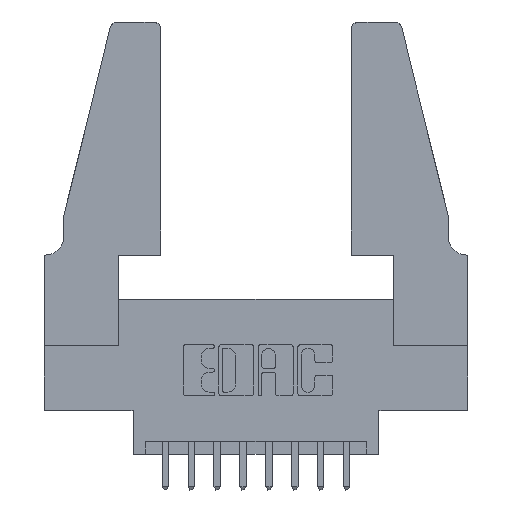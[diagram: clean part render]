
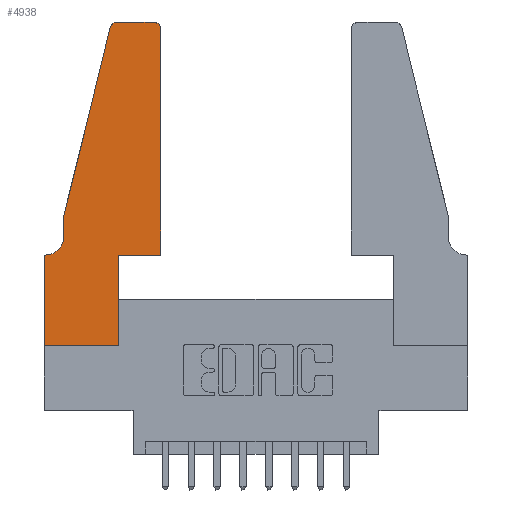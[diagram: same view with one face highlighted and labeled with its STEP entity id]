
A CAD part, top view. The second image highlights one B-rep face of the part: STEP entity #4938.
In plain terms, the highlighted planar face has unit normal (0, 0, 1).
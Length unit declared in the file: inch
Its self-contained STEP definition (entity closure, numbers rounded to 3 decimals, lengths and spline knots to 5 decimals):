
#205 = CARTESIAN_POINT ( 'NONE',  ( 0.284, 1.22, 0.37 ) ) ;
#284 = DIRECTION ( 'NONE',  ( 0., 0., 1. ) ) ;
#294 = EDGE_CURVE ( 'NONE', #1931, #2083, #7622, .T. ) ;
#692 = DIRECTION ( 'NONE',  ( 0., 1., 0. ) ) ;
#739 = CARTESIAN_POINT ( 'NONE',  ( 0.0755, 0.5, 0.37 ) ) ;
#795 = CARTESIAN_POINT ( 'NONE',  ( 0.0755, 0.42, 0.37 ) ) ;
#846 = EDGE_CURVE ( 'NONE', #7038, #6351, #1083, .T. ) ;
#870 = DIRECTION ( 'NONE',  ( 1., 0., 0. ) ) ;
#997 = ORIENTED_EDGE ( 'NONE', *, *, #3256, .T. ) ;
#1051 = CARTESIAN_POINT ( 'NONE',  ( 0.0755, 0.5, 0.37 ) ) ;
#1083 = LINE ( 'NONE', #8374, #8864 ) ;
#1498 = DIRECTION ( 'NONE',  ( 1., 0., 0. ) ) ;
#1621 = DIRECTION ( 'NONE',  ( 0., 0., -1. ) ) ;
#1684 = CARTESIAN_POINT ( 'NONE',  ( 0.0755, 0.35, 0.37 ) ) ;
#1690 = DIRECTION ( 'NONE',  ( 0., -1., 0. ) ) ;
#1698 = DIRECTION ( 'NONE',  ( -1., 0., 0. ) ) ;
#1899 = CIRCLE ( 'NONE', #6041, 0.07 ) ;
#1931 = VERTEX_POINT ( 'NONE', #13122 ) ;
#2083 = VERTEX_POINT ( 'NONE', #4257 ) ;
#2161 = AXIS2_PLACEMENT_3D ( 'NONE', #11984, #6101, #870 ) ;
#2348 = DIRECTION ( 'NONE',  ( 1., 0., 0. ) ) ;
#2449 = CARTESIAN_POINT ( 'NONE',  ( 0.4205, 1.22, 0.37 ) ) ;
#2551 = CARTESIAN_POINT ( 'NONE',  ( 0., 0., 0.37 ) ) ;
#2644 = CARTESIAN_POINT ( 'NONE',  ( 0.0055, 0.42, 0.37 ) ) ;
#2874 = DIRECTION ( 'NONE',  ( -1., 0., 0. ) ) ;
#3157 = VERTEX_POINT ( 'NONE', #10702 ) ;
#3256 = EDGE_CURVE ( 'NONE', #11287, #6496, #10385, .T. ) ;
#3401 = EDGE_LOOP ( 'NONE', ( #11480, #9987, #997, #12524, #6514, #8560, #8275, #5488, #4520, #5731, #10199, #4979 ) ) ;
#3553 = CARTESIAN_POINT ( 'NONE',  ( 0.4505, 0.35, 0.37 ) ) ;
#3646 = EDGE_CURVE ( 'NONE', #5559, #4359, #5180, .T. ) ;
#4061 = PLANE ( 'NONE',  #2161 ) ;
#4157 = EDGE_CURVE ( 'NONE', #4359, #12903, #7979, .T. ) ;
#4257 = CARTESIAN_POINT ( 'NONE',  ( 0., 0.35, 0.37 ) ) ;
#4306 = VECTOR ( 'NONE', #10437, 39.37008 ) ;
#4350 = DIRECTION ( 'NONE',  ( 0., 0., 1. ) ) ;
#4359 = VERTEX_POINT ( 'NONE', #11068 ) ;
#4520 = ORIENTED_EDGE ( 'NONE', *, *, #4157, .T. ) ;
#4556 = LINE ( 'NONE', #1051, #11165 ) ;
#4602 = CARTESIAN_POINT ( 'NONE',  ( 0.4505, 0.35, 0.37 ) ) ;
#4938 = ADVANCED_FACE ( 'NONE', ( #8599 ), #4061, .T. ) ;
#4979 = ORIENTED_EDGE ( 'NONE', *, *, #6165, .T. ) ;
#5180 = LINE ( 'NONE', #11621, #12761 ) ;
#5488 = ORIENTED_EDGE ( 'NONE', *, *, #3646, .T. ) ;
#5559 = VERTEX_POINT ( 'NONE', #2551 ) ;
#5731 = ORIENTED_EDGE ( 'NONE', *, *, #7010, .T. ) ;
#5947 = VECTOR ( 'NONE', #1698, 39.37008 ) ;
#5952 = VECTOR ( 'NONE', #692, 39.37008 ) ;
#6041 = AXIS2_PLACEMENT_3D ( 'NONE', #2644, #1621, #7700 ) ;
#6101 = DIRECTION ( 'NONE',  ( 0., 0., 1. ) ) ;
#6165 = EDGE_CURVE ( 'NONE', #6351, #3157, #9343, .T. ) ;
#6251 = CARTESIAN_POINT ( 'NONE',  ( 0.2865, 0.35, 0.37 ) ) ;
#6351 = VERTEX_POINT ( 'NONE', #12873 ) ;
#6447 = DIRECTION ( 'NONE',  ( 0., -1., 0. ) ) ;
#6496 = VERTEX_POINT ( 'NONE', #13127 ) ;
#6514 = ORIENTED_EDGE ( 'NONE', *, *, #7148, .T. ) ;
#6743 = CARTESIAN_POINT ( 'NONE',  ( 0.284, 1.25, 0.37 ) ) ;
#6774 = CARTESIAN_POINT ( 'NONE',  ( 0.2605, 1.25, 0.37 ) ) ;
#7010 = EDGE_CURVE ( 'NONE', #12903, #7038, #9349, .T. ) ;
#7038 = VERTEX_POINT ( 'NONE', #4602 ) ;
#7148 = EDGE_CURVE ( 'NONE', #10518, #1931, #1899, .T. ) ;
#7197 = LINE ( 'NONE', #6774, #5947 ) ;
#7273 = AXIS2_PLACEMENT_3D ( 'NONE', #2449, #284, #2348 ) ;
#7422 = DIRECTION ( 'NONE',  ( 1., 0., 0. ) ) ;
#7469 = VECTOR ( 'NONE', #2874, 39.37008 ) ;
#7542 = VECTOR ( 'NONE', #8811, 39.37008 ) ;
#7622 = LINE ( 'NONE', #1684, #7469 ) ;
#7700 = DIRECTION ( 'NONE',  ( -1., 0., 0. ) ) ;
#7863 = EDGE_CURVE ( 'NONE', #2083, #5559, #11432, .T. ) ;
#7979 = LINE ( 'NONE', #13042, #5952 ) ;
#8070 = VECTOR ( 'NONE', #1690, 39.37008 ) ;
#8082 = CIRCLE ( 'NONE', #13096, 0.03 ) ;
#8175 = EDGE_CURVE ( 'NONE', #6496, #10518, #4556, .T. ) ;
#8275 = ORIENTED_EDGE ( 'NONE', *, *, #7863, .T. ) ;
#8374 = CARTESIAN_POINT ( 'NONE',  ( 0.4505, 0.35, 0.37 ) ) ;
#8560 = ORIENTED_EDGE ( 'NONE', *, *, #294, .T. ) ;
#8599 = FACE_OUTER_BOUND ( 'NONE', #3401, .T. ) ;
#8692 = CARTESIAN_POINT ( 'NONE',  ( 0., 0., 0.37 ) ) ;
#8811 = DIRECTION ( 'NONE',  ( -0.239, -0.971, 0. ) ) ;
#8864 = VECTOR ( 'NONE', #10014, 39.37008 ) ;
#8895 = EDGE_CURVE ( 'NONE', #3157, #12568, #7197, .T. ) ;
#9343 = CIRCLE ( 'NONE', #7273, 0.03 ) ;
#9349 = LINE ( 'NONE', #3553, #4306 ) ;
#9987 = ORIENTED_EDGE ( 'NONE', *, *, #10200, .T. ) ;
#10014 = DIRECTION ( 'NONE',  ( 0., 1., 0. ) ) ;
#10199 = ORIENTED_EDGE ( 'NONE', *, *, #846, .T. ) ;
#10200 = EDGE_CURVE ( 'NONE', #12568, #11287, #8082, .T. ) ;
#10385 = LINE ( 'NONE', #739, #7542 ) ;
#10437 = DIRECTION ( 'NONE',  ( 1., 0., 0. ) ) ;
#10518 = VERTEX_POINT ( 'NONE', #795 ) ;
#10702 = CARTESIAN_POINT ( 'NONE',  ( 0.4205, 1.25, 0.37 ) ) ;
#11068 = CARTESIAN_POINT ( 'NONE',  ( 0.2865, 0., 0.37 ) ) ;
#11165 = VECTOR ( 'NONE', #6447, 39.37008 ) ;
#11287 = VERTEX_POINT ( 'NONE', #11469 ) ;
#11432 = LINE ( 'NONE', #8692, #8070 ) ;
#11469 = CARTESIAN_POINT ( 'NONE',  ( 0.25487, 1.22718, 0.37 ) ) ;
#11480 = ORIENTED_EDGE ( 'NONE', *, *, #8895, .T. ) ;
#11621 = CARTESIAN_POINT ( 'NONE',  ( 0., 0., 0.37 ) ) ;
#11984 = CARTESIAN_POINT ( 'NONE',  ( 0., 0.35, 0.37 ) ) ;
#12524 = ORIENTED_EDGE ( 'NONE', *, *, #8175, .T. ) ;
#12568 = VERTEX_POINT ( 'NONE', #6743 ) ;
#12761 = VECTOR ( 'NONE', #1498, 39.37008 ) ;
#12873 = CARTESIAN_POINT ( 'NONE',  ( 0.4505, 1.22, 0.37 ) ) ;
#12903 = VERTEX_POINT ( 'NONE', #6251 ) ;
#13042 = CARTESIAN_POINT ( 'NONE',  ( 0.2865, 0.35, 0.37 ) ) ;
#13096 = AXIS2_PLACEMENT_3D ( 'NONE', #205, #4350, #7422 ) ;
#13122 = CARTESIAN_POINT ( 'NONE',  ( 0.0055, 0.35, 0.37 ) ) ;
#13127 = CARTESIAN_POINT ( 'NONE',  ( 0.0755, 0.5, 0.37 ) ) ;
